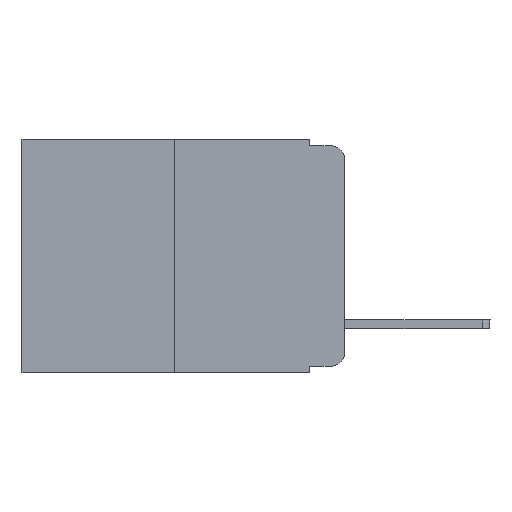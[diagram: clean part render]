
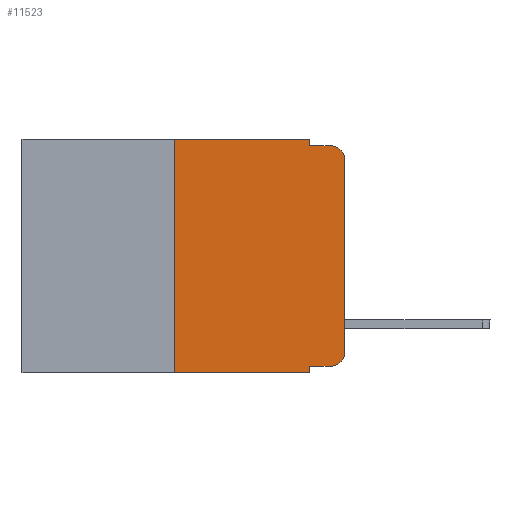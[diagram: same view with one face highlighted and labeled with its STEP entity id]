
A CAD part, left-side view. The second image highlights one B-rep face of the part: STEP entity #11523.
In plain terms, the highlighted planar face has unit normal (-1, 0, 0).
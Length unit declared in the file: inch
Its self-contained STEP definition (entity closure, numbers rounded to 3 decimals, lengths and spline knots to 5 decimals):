
#173 = CARTESIAN_POINT ( 'NONE',  ( 0., 0.473, 0. ) ) ;
#692 = CARTESIAN_POINT ( 'NONE',  ( 0., 0.02, -0.01 ) ) ;
#823 = CARTESIAN_POINT ( 'NONE',  ( 0., 0.25, -0.343 ) ) ;
#994 = CARTESIAN_POINT ( 'NONE',  ( 0., 0.473, -0.343 ) ) ;
#1076 = VECTOR ( 'NONE', #14546, 39.37008 ) ;
#1297 = ORIENTED_EDGE ( 'NONE', *, *, #5736, .T. ) ;
#1673 = CARTESIAN_POINT ( 'NONE',  ( 0., 0., -0.313 ) ) ;
#1943 = VECTOR ( 'NONE', #13558, 39.37008 ) ;
#2065 = CARTESIAN_POINT ( 'NONE',  ( 0., 0.051, -0.01 ) ) ;
#2072 = ORIENTED_EDGE ( 'NONE', *, *, #11193, .T. ) ;
#2182 = AXIS2_PLACEMENT_3D ( 'NONE', #173, #9951, #11683 ) ;
#2336 = DIRECTION ( 'NONE',  ( 0., -1., 0. ) ) ;
#2426 = CARTESIAN_POINT ( 'NONE',  ( 0., 0.473, 0. ) ) ;
#2436 = LINE ( 'NONE', #6649, #1943 ) ;
#2481 = DIRECTION ( 'NONE',  ( 0., 0., -1. ) ) ;
#2524 = VECTOR ( 'NONE', #2336, 39.37008 ) ;
#2669 = DIRECTION ( 'NONE',  ( 0., 0., 1. ) ) ;
#2696 = CARTESIAN_POINT ( 'NONE',  ( 0., 0.25, 0. ) ) ;
#2769 = VERTEX_POINT ( 'NONE', #692 ) ;
#2927 = LINE ( 'NONE', #14152, #15053 ) ;
#3122 = EDGE_CURVE ( 'NONE', #13850, #2769, #11354, .T. ) ;
#3125 = CARTESIAN_POINT ( 'NONE',  ( 0., 0.02, -0.03 ) ) ;
#3490 = AXIS2_PLACEMENT_3D ( 'NONE', #3125, #14169, #17268 ) ;
#3639 = CARTESIAN_POINT ( 'NONE',  ( 0., 0.051, 0. ) ) ;
#3665 = EDGE_CURVE ( 'NONE', #12169, #2769, #2436, .T. ) ;
#3741 = LINE ( 'NONE', #994, #8787 ) ;
#3759 = VERTEX_POINT ( 'NONE', #2696 ) ;
#3952 = LINE ( 'NONE', #8251, #10550 ) ;
#4110 = VECTOR ( 'NONE', #16858, 39.37008 ) ;
#4583 = DIRECTION ( 'NONE',  ( 0., 0., -1. ) ) ;
#4938 = EDGE_CURVE ( 'NONE', #7861, #14698, #3741, .T. ) ;
#5028 = ORIENTED_EDGE ( 'NONE', *, *, #4938, .T. ) ;
#5143 = EDGE_CURVE ( 'NONE', #13486, #14698, #8670, .T. ) ;
#5418 = CARTESIAN_POINT ( 'NONE',  ( 0., 0.25, 0. ) ) ;
#5532 = CARTESIAN_POINT ( 'NONE',  ( 0., 0.051, -0.333 ) ) ;
#5736 = EDGE_CURVE ( 'NONE', #14353, #11016, #5838, .T. ) ;
#5838 = CIRCLE ( 'NONE', #16018, 0.02 ) ;
#5974 = LINE ( 'NONE', #12908, #1076 ) ;
#6546 = ORIENTED_EDGE ( 'NONE', *, *, #5143, .F. ) ;
#6649 = CARTESIAN_POINT ( 'NONE',  ( 0., 0.051, -0.01 ) ) ;
#7433 = ORIENTED_EDGE ( 'NONE', *, *, #10862, .F. ) ;
#7861 = VERTEX_POINT ( 'NONE', #823 ) ;
#8251 = CARTESIAN_POINT ( 'NONE',  ( 0., 0., 0. ) ) ;
#8503 = FACE_OUTER_BOUND ( 'NONE', #11008, .T. ) ;
#8670 = LINE ( 'NONE', #10310, #4110 ) ;
#8787 = VECTOR ( 'NONE', #10775, 39.37008 ) ;
#9841 = CARTESIAN_POINT ( 'NONE',  ( 0., 0.02, -0.333 ) ) ;
#9951 = DIRECTION ( 'NONE',  ( 1., 0., 0. ) ) ;
#10168 = ORIENTED_EDGE ( 'NONE', *, *, #14806, .F. ) ;
#10222 = PLANE ( 'NONE',  #2182 ) ;
#10310 = CARTESIAN_POINT ( 'NONE',  ( 0., 0.051, 0. ) ) ;
#10383 = VERTEX_POINT ( 'NONE', #3639 ) ;
#10550 = VECTOR ( 'NONE', #16441, 39.37008 ) ;
#10775 = DIRECTION ( 'NONE',  ( 0., -1., 0. ) ) ;
#10862 = EDGE_CURVE ( 'NONE', #3759, #10383, #14567, .T. ) ;
#11008 = EDGE_LOOP ( 'NONE', ( #17318, #13231, #13919, #10168, #7433, #16588, #5028, #6546, #2072, #1297 ) ) ;
#11016 = VERTEX_POINT ( 'NONE', #1673 ) ;
#11193 = EDGE_CURVE ( 'NONE', #13486, #14353, #5974, .T. ) ;
#11354 = CIRCLE ( 'NONE', #3490, 0.02 ) ;
#11523 = ADVANCED_FACE ( 'NONE', ( #8503 ), #10222, .F. ) ;
#11683 = DIRECTION ( 'NONE',  ( 0., 0., -1. ) ) ;
#12169 = VERTEX_POINT ( 'NONE', #2065 ) ;
#12338 = CARTESIAN_POINT ( 'NONE',  ( 0., 0.051, -0.343 ) ) ;
#12640 = EDGE_CURVE ( 'NONE', #7861, #3759, #15166, .T. ) ;
#12908 = CARTESIAN_POINT ( 'NONE',  ( 0., 0.051, -0.333 ) ) ;
#13231 = ORIENTED_EDGE ( 'NONE', *, *, #3122, .T. ) ;
#13486 = VERTEX_POINT ( 'NONE', #5532 ) ;
#13558 = DIRECTION ( 'NONE',  ( 0., -1., 0. ) ) ;
#13850 = VERTEX_POINT ( 'NONE', #14461 ) ;
#13919 = ORIENTED_EDGE ( 'NONE', *, *, #3665, .F. ) ;
#14083 = VECTOR ( 'NONE', #2669, 39.37008 ) ;
#14152 = CARTESIAN_POINT ( 'NONE',  ( 0., 0.051, 0. ) ) ;
#14169 = DIRECTION ( 'NONE',  ( -1., 0., 0. ) ) ;
#14353 = VERTEX_POINT ( 'NONE', #9841 ) ;
#14461 = CARTESIAN_POINT ( 'NONE',  ( 0., 0., -0.03 ) ) ;
#14546 = DIRECTION ( 'NONE',  ( 0., -1., 0. ) ) ;
#14567 = LINE ( 'NONE', #2426, #2524 ) ;
#14698 = VERTEX_POINT ( 'NONE', #12338 ) ;
#14806 = EDGE_CURVE ( 'NONE', #10383, #12169, #2927, .T. ) ;
#15053 = VECTOR ( 'NONE', #4583, 39.37008 ) ;
#15166 = LINE ( 'NONE', #5418, #14083 ) ;
#16018 = AXIS2_PLACEMENT_3D ( 'NONE', #17454, #16431, #2481 ) ;
#16431 = DIRECTION ( 'NONE',  ( -1., 0., 0. ) ) ;
#16441 = DIRECTION ( 'NONE',  ( 0., 0., 1. ) ) ;
#16588 = ORIENTED_EDGE ( 'NONE', *, *, #12640, .F. ) ;
#16858 = DIRECTION ( 'NONE',  ( 0., 0., -1. ) ) ;
#17268 = DIRECTION ( 'NONE',  ( 0., 0., -1. ) ) ;
#17318 = ORIENTED_EDGE ( 'NONE', *, *, #17675, .T. ) ;
#17454 = CARTESIAN_POINT ( 'NONE',  ( 0., 0.02, -0.313 ) ) ;
#17675 = EDGE_CURVE ( 'NONE', #11016, #13850, #3952, .T. ) ;
